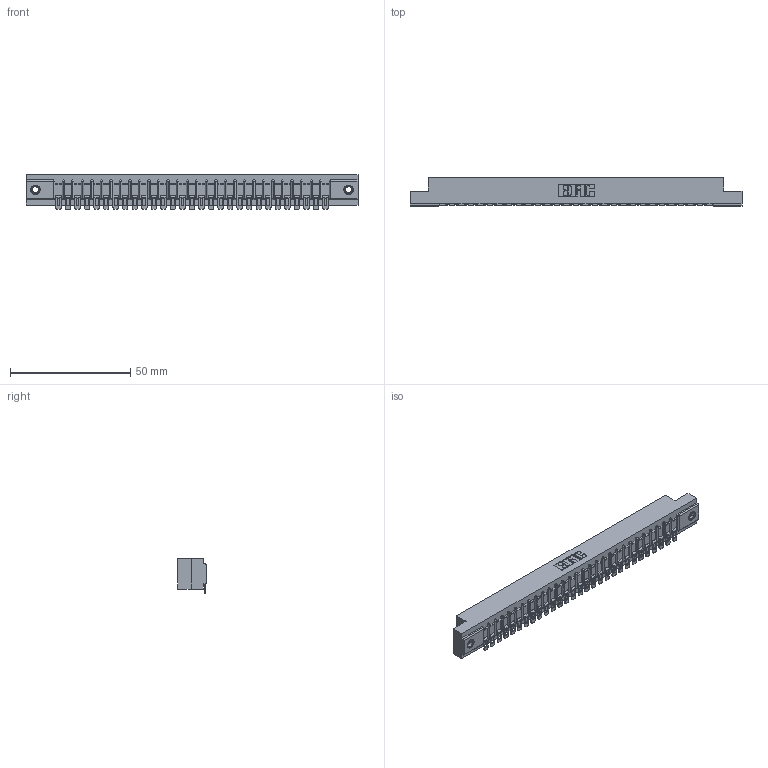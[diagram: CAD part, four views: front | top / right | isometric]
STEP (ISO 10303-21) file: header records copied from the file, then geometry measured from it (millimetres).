
FILE_DESCRIPTION (( 'STEP AP203' ), '1' );
FILE_NAME ('307-029-554-107.STEP', '2018-08-04T18:10:11', ( '' ), ( '' ), 'SwSTEP 2.0', 'SolidWorks 2016', '' );
FILE_SCHEMA (( 'CONFIG_CONTROL_DESIGN' ));
Length unit declared in the file: inch
Products named in the file (4): 307 Part_.156 Dia Mounting Holes; 307-290-002_554; 345-250-001_345-250-005-103; 307-029-554-107
Assembly tree (32 placements, depth 2):
  307-029-554-107
    307 Part_.156 Dia Mounting Holes
    307-290-002_554  x29
    345-250-001_345-250-005-103  x2
Bounding box: 137.92 x 12.01 x 14.52 mm (x, y, z)
Volume: 14659.4 mm3; surface area: 18291.8 mm2
Topology: 32 solids, 32 shells, 2557 faces, 7796 edges, 5108 vertices
Faces by surface type: plane 1436, cylinder 1045, sphere 60, cone 12, torus 4
Entity records: 28614 total; most frequent: CARTESIAN_POINT 4805, ORIENTED_EDGE 4788, DIRECTION 4690, EDGE_CURVE 2394, LINE 1820, VECTOR 1820, VERTEX_POINT 1550, AXIS2_PLACEMENT_3D 1435
